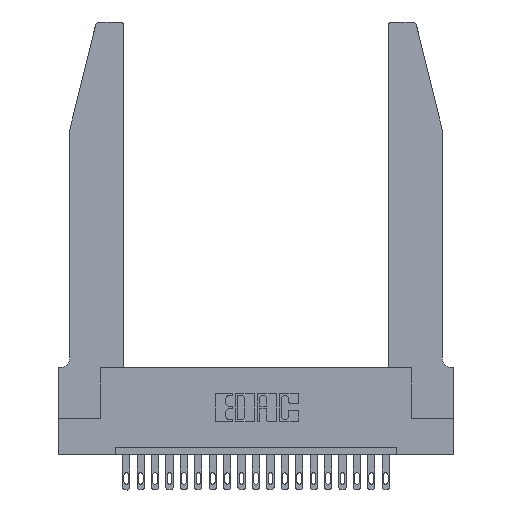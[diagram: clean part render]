
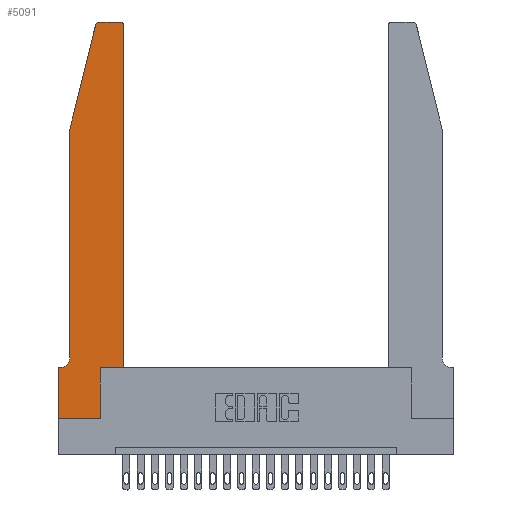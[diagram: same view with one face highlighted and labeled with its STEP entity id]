
A CAD part, top view. The second image highlights one B-rep face of the part: STEP entity #5091.
In plain terms, the highlighted planar face has unit normal (0, 0, 1).
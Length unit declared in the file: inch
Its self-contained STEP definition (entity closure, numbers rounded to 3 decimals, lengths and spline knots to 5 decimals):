
#12 = CARTESIAN_POINT ( 'NONE',  ( 0.0755, 0.42, 0.37 ) ) ;
#270 = CARTESIAN_POINT ( 'NONE',  ( 0.0755, 0.35, 0.37 ) ) ;
#409 = DIRECTION ( 'NONE',  ( 1., 0., 0. ) ) ;
#429 = DIRECTION ( 'NONE',  ( 0., -1., 0. ) ) ;
#664 = CIRCLE ( 'NONE', #4830, 0.03 ) ;
#1199 = ORIENTED_EDGE ( 'NONE', *, *, #6282, .T. ) ;
#1342 = CARTESIAN_POINT ( 'NONE',  ( 0., 0.35, 0.37 ) ) ;
#1460 = VECTOR ( 'NONE', #429, 39.37008 ) ;
#1468 = CARTESIAN_POINT ( 'NONE',  ( 0.284, 2.75, 0.37 ) ) ;
#1480 = VERTEX_POINT ( 'NONE', #2167 ) ;
#1710 = CARTESIAN_POINT ( 'NONE',  ( 0.4505, 0.35, 0.37 ) ) ;
#1849 = LINE ( 'NONE', #20374, #18140 ) ;
#1940 = CARTESIAN_POINT ( 'NONE',  ( 0.2865, 0.35, 0.37 ) ) ;
#2167 = CARTESIAN_POINT ( 'NONE',  ( 0.2865, 0., 0.37 ) ) ;
#2203 = VERTEX_POINT ( 'NONE', #4132 ) ;
#2621 = ORIENTED_EDGE ( 'NONE', *, *, #15403, .T. ) ;
#3007 = EDGE_CURVE ( 'NONE', #12459, #1480, #19757, .T. ) ;
#3069 = CARTESIAN_POINT ( 'NONE',  ( 0.0755, 2., 0.37 ) ) ;
#3100 = ORIENTED_EDGE ( 'NONE', *, *, #20338, .T. ) ;
#3386 = FACE_OUTER_BOUND ( 'NONE', #5285, .T. ) ;
#3408 = AXIS2_PLACEMENT_3D ( 'NONE', #1342, #13330, #8372 ) ;
#3736 = EDGE_CURVE ( 'NONE', #6797, #20016, #1849, .T. ) ;
#3817 = DIRECTION ( 'NONE',  ( 0., 0., 1. ) ) ;
#3908 = DIRECTION ( 'NONE',  ( -1., 0., 0. ) ) ;
#4032 = DIRECTION ( 'NONE',  ( 0., 0., 1. ) ) ;
#4132 = CARTESIAN_POINT ( 'NONE',  ( 0.0055, 0.35, 0.37 ) ) ;
#4393 = VERTEX_POINT ( 'NONE', #1710 ) ;
#4830 = AXIS2_PLACEMENT_3D ( 'NONE', #10240, #4032, #19284 ) ;
#5091 = ADVANCED_FACE ( 'NONE', ( #3386 ), #18355, .T. ) ;
#5285 = EDGE_LOOP ( 'NONE', ( #12084, #1199, #17855, #20367, #14227, #19461, #9452, #20260, #13039, #3100, #18655, #2621 ) ) ;
#5333 = CARTESIAN_POINT ( 'NONE',  ( 0.4505, 0.35, 0.37 ) ) ;
#6162 = CARTESIAN_POINT ( 'NONE',  ( 0., 0., 0.37 ) ) ;
#6282 = EDGE_CURVE ( 'NONE', #20016, #14645, #664, .T. ) ;
#6441 = VECTOR ( 'NONE', #17239, 39.37008 ) ;
#6706 = LINE ( 'NONE', #17030, #6441 ) ;
#6797 = VERTEX_POINT ( 'NONE', #15763 ) ;
#6929 = CARTESIAN_POINT ( 'NONE',  ( 0.4205, 2.72, 0.37 ) ) ;
#7058 = EDGE_CURVE ( 'NONE', #14645, #18824, #18260, .T. ) ;
#7124 = LINE ( 'NONE', #13331, #14025 ) ;
#7254 = VECTOR ( 'NONE', #21000, 39.37008 ) ;
#7656 = DIRECTION ( 'NONE',  ( -1., 0., 0. ) ) ;
#7775 = VECTOR ( 'NONE', #11211, 39.37008 ) ;
#7855 = VERTEX_POINT ( 'NONE', #19878 ) ;
#8206 = EDGE_CURVE ( 'NONE', #12159, #2203, #19014, .T. ) ;
#8372 = DIRECTION ( 'NONE',  ( 1., 0., 0. ) ) ;
#9072 = CARTESIAN_POINT ( 'NONE',  ( 0.4505, 0.35, 0.37 ) ) ;
#9452 = ORIENTED_EDGE ( 'NONE', *, *, #9733, .T. ) ;
#9733 = EDGE_CURVE ( 'NONE', #20688, #12459, #19360, .T. ) ;
#10240 = CARTESIAN_POINT ( 'NONE',  ( 0.284, 2.72, 0.37 ) ) ;
#11211 = DIRECTION ( 'NONE',  ( 1., 0., 0. ) ) ;
#11263 = CARTESIAN_POINT ( 'NONE',  ( 0.0055, 0.42, 0.37 ) ) ;
#11463 = EDGE_CURVE ( 'NONE', #4393, #7855, #14199, .T. ) ;
#11836 = DIRECTION ( 'NONE',  ( 0., -1., 0. ) ) ;
#12084 = ORIENTED_EDGE ( 'NONE', *, *, #3736, .T. ) ;
#12143 = EDGE_CURVE ( 'NONE', #1480, #16615, #6706, .T. ) ;
#12159 = VERTEX_POINT ( 'NONE', #12 ) ;
#12459 = VERTEX_POINT ( 'NONE', #17894 ) ;
#12940 = CIRCLE ( 'NONE', #13779, 0.03 ) ;
#13039 = ORIENTED_EDGE ( 'NONE', *, *, #12143, .T. ) ;
#13330 = DIRECTION ( 'NONE',  ( 0., 0., 1. ) ) ;
#13331 = CARTESIAN_POINT ( 'NONE',  ( 0.0755, 2., 0.37 ) ) ;
#13447 = LINE ( 'NONE', #270, #17462 ) ;
#13779 = AXIS2_PLACEMENT_3D ( 'NONE', #6929, #3817, #409 ) ;
#14025 = VECTOR ( 'NONE', #11836, 39.37008 ) ;
#14199 = LINE ( 'NONE', #5333, #18989 ) ;
#14227 = ORIENTED_EDGE ( 'NONE', *, *, #8206, .T. ) ;
#14297 = DIRECTION ( 'NONE',  ( 0., 1., 0. ) ) ;
#14423 = DIRECTION ( 'NONE',  ( -0.239, -0.971, 0. ) ) ;
#14645 = VERTEX_POINT ( 'NONE', #21988 ) ;
#14655 = EDGE_CURVE ( 'NONE', #18824, #12159, #7124, .T. ) ;
#15257 = DIRECTION ( 'NONE',  ( -1., 0., 0. ) ) ;
#15403 = EDGE_CURVE ( 'NONE', #7855, #6797, #12940, .T. ) ;
#15763 = CARTESIAN_POINT ( 'NONE',  ( 0.4205, 2.75, 0.37 ) ) ;
#16136 = DIRECTION ( 'NONE',  ( 0., 0., -1. ) ) ;
#16347 = LINE ( 'NONE', #9072, #7254 ) ;
#16615 = VERTEX_POINT ( 'NONE', #1940 ) ;
#17030 = CARTESIAN_POINT ( 'NONE',  ( 0.2865, 0.35, 0.37 ) ) ;
#17239 = DIRECTION ( 'NONE',  ( 0., 1., 0. ) ) ;
#17303 = AXIS2_PLACEMENT_3D ( 'NONE', #11263, #16136, #7656 ) ;
#17462 = VECTOR ( 'NONE', #3908, 39.37008 ) ;
#17855 = ORIENTED_EDGE ( 'NONE', *, *, #7058, .T. ) ;
#17894 = CARTESIAN_POINT ( 'NONE',  ( 0., 0., 0.37 ) ) ;
#18140 = VECTOR ( 'NONE', #15257, 39.37008 ) ;
#18260 = LINE ( 'NONE', #21499, #21704 ) ;
#18355 = PLANE ( 'NONE',  #3408 ) ;
#18399 = EDGE_CURVE ( 'NONE', #2203, #20688, #13447, .T. ) ;
#18655 = ORIENTED_EDGE ( 'NONE', *, *, #11463, .T. ) ;
#18824 = VERTEX_POINT ( 'NONE', #3069 ) ;
#18989 = VECTOR ( 'NONE', #14297, 39.37008 ) ;
#19014 = CIRCLE ( 'NONE', #17303, 0.07 ) ;
#19284 = DIRECTION ( 'NONE',  ( 1., 0., 0. ) ) ;
#19360 = LINE ( 'NONE', #22056, #1460 ) ;
#19461 = ORIENTED_EDGE ( 'NONE', *, *, #18399, .T. ) ;
#19757 = LINE ( 'NONE', #6162, #7775 ) ;
#19878 = CARTESIAN_POINT ( 'NONE',  ( 0.4505, 2.72, 0.37 ) ) ;
#20016 = VERTEX_POINT ( 'NONE', #1468 ) ;
#20193 = CARTESIAN_POINT ( 'NONE',  ( 0., 0.35, 0.37 ) ) ;
#20260 = ORIENTED_EDGE ( 'NONE', *, *, #3007, .T. ) ;
#20338 = EDGE_CURVE ( 'NONE', #16615, #4393, #16347, .T. ) ;
#20367 = ORIENTED_EDGE ( 'NONE', *, *, #14655, .T. ) ;
#20374 = CARTESIAN_POINT ( 'NONE',  ( 0.2605, 2.75, 0.37 ) ) ;
#20688 = VERTEX_POINT ( 'NONE', #20193 ) ;
#21000 = DIRECTION ( 'NONE',  ( 1., 0., 0. ) ) ;
#21499 = CARTESIAN_POINT ( 'NONE',  ( 0.0755, 2., 0.37 ) ) ;
#21704 = VECTOR ( 'NONE', #14423, 39.37008 ) ;
#21988 = CARTESIAN_POINT ( 'NONE',  ( 0.25487, 2.72718, 0.37 ) ) ;
#22056 = CARTESIAN_POINT ( 'NONE',  ( 0., 0., 0.37 ) ) ;
